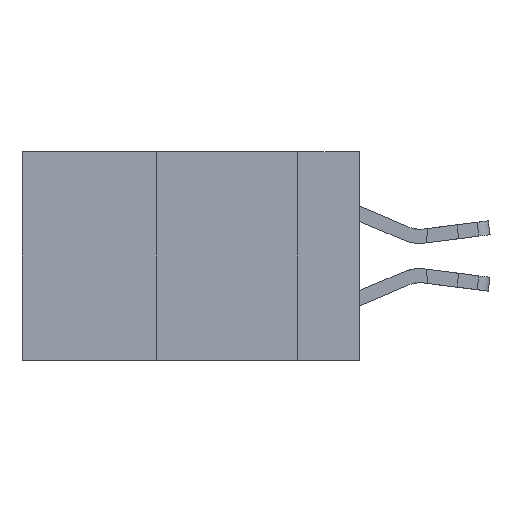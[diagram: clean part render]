
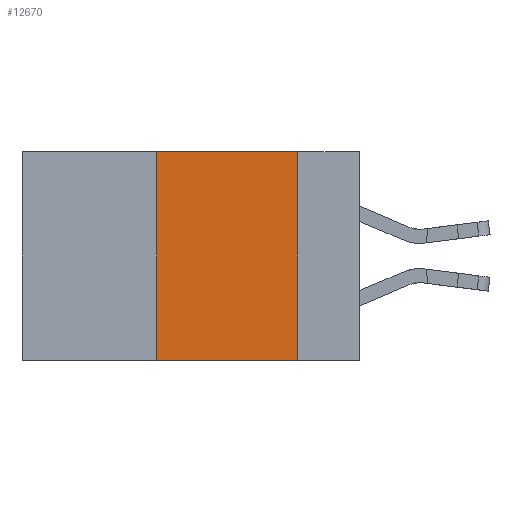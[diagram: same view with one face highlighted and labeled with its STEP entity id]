
A CAD part, left-side view. The second image highlights one B-rep face of the part: STEP entity #12670.
In plain terms, the highlighted planar face has unit normal (-1, 0, 0).
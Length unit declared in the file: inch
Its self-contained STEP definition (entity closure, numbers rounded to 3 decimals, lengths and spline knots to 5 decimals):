
#273 = VECTOR ( 'NONE', #16746, 39.37008 ) ;
#456 = ORIENTED_EDGE ( 'NONE', *, *, #4026, .F. ) ;
#595 = VECTOR ( 'NONE', #18810, 39.37008 ) ;
#1031 = EDGE_CURVE ( 'NONE', #5543, #12933, #18973, .T. ) ;
#1314 = ORIENTED_EDGE ( 'NONE', *, *, #1031, .T. ) ;
#2049 = CARTESIAN_POINT ( 'NONE',  ( 0., 0.6, -0.37 ) ) ;
#2780 = PLANE ( 'NONE',  #5367 ) ;
#2903 = EDGE_CURVE ( 'NONE', #3155, #12933, #17194, .T. ) ;
#3155 = VERTEX_POINT ( 'NONE', #12317 ) ;
#4026 = EDGE_CURVE ( 'NONE', #20087, #3155, #11364, .T. ) ;
#5367 = AXIS2_PLACEMENT_3D ( 'NONE', #17908, #9574, #21130 ) ;
#5543 = VERTEX_POINT ( 'NONE', #20184 ) ;
#6522 = FACE_OUTER_BOUND ( 'NONE', #8002, .T. ) ;
#6816 = EDGE_CURVE ( 'NONE', #5543, #20087, #21289, .T. ) ;
#8002 = EDGE_LOOP ( 'NONE', ( #17875, #456, #20874, #1314 ) ) ;
#9574 = DIRECTION ( 'NONE',  ( 1., 0., 0. ) ) ;
#11364 = LINE ( 'NONE', #16601, #19657 ) ;
#12317 = CARTESIAN_POINT ( 'NONE',  ( 0., 0.11, 0. ) ) ;
#12521 = DIRECTION ( 'NONE',  ( 0., 0., 1. ) ) ;
#12670 = ADVANCED_FACE ( 'NONE', ( #6522 ), #2780, .F. ) ;
#12933 = VERTEX_POINT ( 'NONE', #20963 ) ;
#13380 = CARTESIAN_POINT ( 'NONE',  ( 0., 0.11, 0. ) ) ;
#14164 = CARTESIAN_POINT ( 'NONE',  ( 0., 0.36, 0. ) ) ;
#16145 = CARTESIAN_POINT ( 'NONE',  ( 0., 0.36, 0. ) ) ;
#16601 = CARTESIAN_POINT ( 'NONE',  ( 0., 0.6, 0. ) ) ;
#16746 = DIRECTION ( 'NONE',  ( 0., 0., -1. ) ) ;
#17029 = VECTOR ( 'NONE', #12521, 39.37008 ) ;
#17194 = LINE ( 'NONE', #13380, #273 ) ;
#17875 = ORIENTED_EDGE ( 'NONE', *, *, #2903, .F. ) ;
#17908 = CARTESIAN_POINT ( 'NONE',  ( 0., 0.6, 0. ) ) ;
#18205 = DIRECTION ( 'NONE',  ( 0., -1., 0. ) ) ;
#18810 = DIRECTION ( 'NONE',  ( 0., -1., 0. ) ) ;
#18973 = LINE ( 'NONE', #2049, #595 ) ;
#19657 = VECTOR ( 'NONE', #18205, 39.37008 ) ;
#20087 = VERTEX_POINT ( 'NONE', #16145 ) ;
#20184 = CARTESIAN_POINT ( 'NONE',  ( 0., 0.36, -0.37 ) ) ;
#20874 = ORIENTED_EDGE ( 'NONE', *, *, #6816, .F. ) ;
#20963 = CARTESIAN_POINT ( 'NONE',  ( 0., 0.11, -0.37 ) ) ;
#21130 = DIRECTION ( 'NONE',  ( 0., 0., -1. ) ) ;
#21289 = LINE ( 'NONE', #14164, #17029 ) ;
